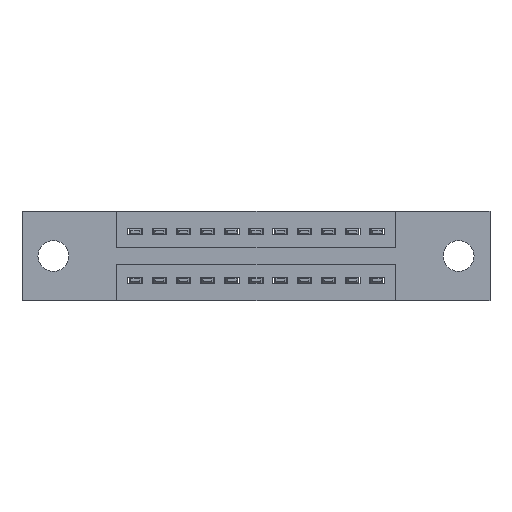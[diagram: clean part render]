
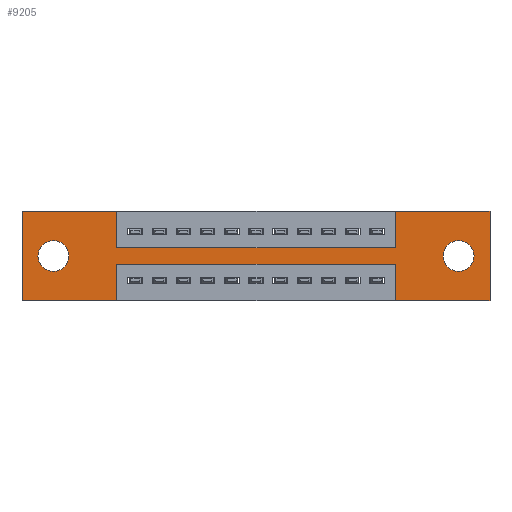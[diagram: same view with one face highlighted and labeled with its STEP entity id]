
A CAD part, front view. The second image highlights one B-rep face of the part: STEP entity #9205.
In plain terms, the highlighted planar face has unit normal (0, -1, 0).
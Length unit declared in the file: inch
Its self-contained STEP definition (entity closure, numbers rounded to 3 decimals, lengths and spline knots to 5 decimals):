
#7 = ORIENTED_EDGE ( 'NONE', *, *, #1507, .F. ) ;
#96 = CARTESIAN_POINT ( 'NONE',  ( 1.5425, 0., -0.15 ) ) ;
#225 = DIRECTION ( 'NONE',  ( 0., 0., 1. ) ) ;
#337 = ORIENTED_EDGE ( 'NONE', *, *, #2822, .F. ) ;
#346 = VECTOR ( 'NONE', #6573, 39.37008 ) ;
#505 = VERTEX_POINT ( 'NONE', #96 ) ;
#539 = VERTEX_POINT ( 'NONE', #2170 ) ;
#620 = FACE_BOUND ( 'NONE', #1701, .T. ) ;
#714 = EDGE_CURVE ( 'NONE', #5986, #6882, #4839, .T. ) ;
#729 = CARTESIAN_POINT ( 'NONE',  ( 0.3925, 0., -0.22 ) ) ;
#983 = CIRCLE ( 'NONE', #7035, 0.064 ) ;
#1058 = CARTESIAN_POINT ( 'NONE',  ( 0.13, 0., -0.121 ) ) ;
#1203 = EDGE_CURVE ( 'NONE', #8654, #8650, #11434, .T. ) ;
#1286 = LINE ( 'NONE', #7946, #9013 ) ;
#1308 = CARTESIAN_POINT ( 'NONE',  ( 0., 0., 0. ) ) ;
#1486 = ORIENTED_EDGE ( 'NONE', *, *, #12150, .T. ) ;
#1507 = EDGE_CURVE ( 'NONE', #6882, #12163, #9912, .T. ) ;
#1580 = LINE ( 'NONE', #7651, #9550 ) ;
#1701 = EDGE_LOOP ( 'NONE', ( #8888, #11293 ) ) ;
#1753 = DIRECTION ( 'NONE',  ( 0., 0., -1. ) ) ;
#1786 = DIRECTION ( 'NONE',  ( 0., 1., 0. ) ) ;
#1807 = ORIENTED_EDGE ( 'NONE', *, *, #4567, .F. ) ;
#1813 = CARTESIAN_POINT ( 'NONE',  ( 1.805, 0., -0.185 ) ) ;
#1900 = LINE ( 'NONE', #4996, #11638 ) ;
#2051 = EDGE_CURVE ( 'NONE', #10428, #4783, #983, .T. ) ;
#2081 = PLANE ( 'NONE',  #5947 ) ;
#2170 = CARTESIAN_POINT ( 'NONE',  ( 1.935, 0., -0.37 ) ) ;
#2176 = CARTESIAN_POINT ( 'NONE',  ( 0., 0., 0. ) ) ;
#2319 = EDGE_CURVE ( 'NONE', #4783, #10428, #12520, .T. ) ;
#2371 = VERTEX_POINT ( 'NONE', #729 ) ;
#2412 = DIRECTION ( 'NONE',  ( 0., 0., -1. ) ) ;
#2484 = ORIENTED_EDGE ( 'NONE', *, *, #10534, .F. ) ;
#2776 = DIRECTION ( 'NONE',  ( 1., 0., 0. ) ) ;
#2822 = EDGE_CURVE ( 'NONE', #8650, #5986, #1286, .T. ) ;
#3068 = VERTEX_POINT ( 'NONE', #11318 ) ;
#3094 = DIRECTION ( 'NONE',  ( 0., 0., -1. ) ) ;
#3098 = ORIENTED_EDGE ( 'NONE', *, *, #1203, .F. ) ;
#3137 = AXIS2_PLACEMENT_3D ( 'NONE', #1813, #1786, #1753 ) ;
#3365 = FACE_OUTER_BOUND ( 'NONE', #4482, .T. ) ;
#3440 = LINE ( 'NONE', #6482, #6171 ) ;
#3688 = VECTOR ( 'NONE', #7209, 39.37008 ) ;
#3947 = EDGE_CURVE ( 'NONE', #7504, #2371, #1580, .T. ) ;
#4091 = DIRECTION ( 'NONE',  ( 1., 0., 0. ) ) ;
#4112 = CIRCLE ( 'NONE', #5354, 0.064 ) ;
#4198 = EDGE_CURVE ( 'NONE', #11257, #7093, #8990, .T. ) ;
#4236 = ORIENTED_EDGE ( 'NONE', *, *, #4198, .T. ) ;
#4347 = CARTESIAN_POINT ( 'NONE',  ( 0.3925, 0., -0.15 ) ) ;
#4482 = EDGE_LOOP ( 'NONE', ( #1807, #7203, #9763, #12130, #7502, #10056, #2484, #5185, #7, #8135, #337, #3098 ) ) ;
#4567 = EDGE_CURVE ( 'NONE', #2371, #8654, #12482, .T. ) ;
#4783 = VERTEX_POINT ( 'NONE', #8374 ) ;
#4839 = LINE ( 'NONE', #8570, #9743 ) ;
#4959 = VECTOR ( 'NONE', #10733, 39.37008 ) ;
#4996 = CARTESIAN_POINT ( 'NONE',  ( 1.5425, 0., 0. ) ) ;
#4997 = VECTOR ( 'NONE', #11927, 39.37008 ) ;
#5185 = ORIENTED_EDGE ( 'NONE', *, *, #11343, .F. ) ;
#5297 = CARTESIAN_POINT ( 'NONE',  ( 0.3925, 0., -0.37 ) ) ;
#5317 = LINE ( 'NONE', #9259, #4997 ) ;
#5354 = AXIS2_PLACEMENT_3D ( 'NONE', #11976, #6372, #225 ) ;
#5770 = CARTESIAN_POINT ( 'NONE',  ( 1.5425, 0., -0.22 ) ) ;
#5947 = AXIS2_PLACEMENT_3D ( 'NONE', #6132, #9085, #3094 ) ;
#5986 = VERTEX_POINT ( 'NONE', #1308 ) ;
#6001 = CARTESIAN_POINT ( 'NONE',  ( 0.13, 0., -0.249 ) ) ;
#6037 = EDGE_CURVE ( 'NONE', #3068, #539, #9807, .T. ) ;
#6096 = FACE_BOUND ( 'NONE', #10351, .T. ) ;
#6132 = CARTESIAN_POINT ( 'NONE',  ( 0., 0., -0.37 ) ) ;
#6171 = VECTOR ( 'NONE', #11282, 39.37008 ) ;
#6372 = DIRECTION ( 'NONE',  ( 0., 1., 0. ) ) ;
#6482 = CARTESIAN_POINT ( 'NONE',  ( 1.5425, 0., -0.37 ) ) ;
#6573 = DIRECTION ( 'NONE',  ( -1., 0., 0. ) ) ;
#6882 = VERTEX_POINT ( 'NONE', #10654 ) ;
#7035 = AXIS2_PLACEMENT_3D ( 'NONE', #11490, #11443, #11372 ) ;
#7093 = VERTEX_POINT ( 'NONE', #1058 ) ;
#7203 = ORIENTED_EDGE ( 'NONE', *, *, #3947, .F. ) ;
#7209 = DIRECTION ( 'NONE',  ( 1., 0., 0. ) ) ;
#7250 = VECTOR ( 'NONE', #8480, 39.37008 ) ;
#7328 = CARTESIAN_POINT ( 'NONE',  ( 0.3925, 0., 0. ) ) ;
#7463 = CARTESIAN_POINT ( 'NONE',  ( 1.935, 0., 0. ) ) ;
#7502 = ORIENTED_EDGE ( 'NONE', *, *, #6037, .F. ) ;
#7504 = VERTEX_POINT ( 'NONE', #5770 ) ;
#7651 = CARTESIAN_POINT ( 'NONE',  ( 0.3925, 0., -0.22 ) ) ;
#7710 = DIRECTION ( 'NONE',  ( -1., 0., 0. ) ) ;
#7900 = EDGE_CURVE ( 'NONE', #539, #9776, #5317, .T. ) ;
#7946 = CARTESIAN_POINT ( 'NONE',  ( 0., 0., 0. ) ) ;
#8085 = LINE ( 'NONE', #2176, #3688 ) ;
#8135 = ORIENTED_EDGE ( 'NONE', *, *, #714, .F. ) ;
#8374 = CARTESIAN_POINT ( 'NONE',  ( 1.805, 0., -0.249 ) ) ;
#8480 = DIRECTION ( 'NONE',  ( 0., 0., -1. ) ) ;
#8570 = CARTESIAN_POINT ( 'NONE',  ( 0., 0., 0. ) ) ;
#8598 = EDGE_CURVE ( 'NONE', #10184, #3068, #8085, .T. ) ;
#8650 = VERTEX_POINT ( 'NONE', #11011 ) ;
#8654 = VERTEX_POINT ( 'NONE', #5297 ) ;
#8778 = CARTESIAN_POINT ( 'NONE',  ( 1.5425, 0., -0.37 ) ) ;
#8888 = ORIENTED_EDGE ( 'NONE', *, *, #2051, .T. ) ;
#8942 = AXIS2_PLACEMENT_3D ( 'NONE', #12438, #12423, #12398 ) ;
#8990 = CIRCLE ( 'NONE', #8942, 0.064 ) ;
#9013 = VECTOR ( 'NONE', #11468, 39.37008 ) ;
#9042 = CARTESIAN_POINT ( 'NONE',  ( 0.3925, 0., -0.15 ) ) ;
#9085 = DIRECTION ( 'NONE',  ( 0., -1., 0. ) ) ;
#9205 = ADVANCED_FACE ( 'NONE', ( #620, #6096, #3365 ), #2081, .T. ) ;
#9259 = CARTESIAN_POINT ( 'NONE',  ( 0., 0., -0.37 ) ) ;
#9310 = CARTESIAN_POINT ( 'NONE',  ( 0., 0., -0.37 ) ) ;
#9384 = CARTESIAN_POINT ( 'NONE',  ( 1.5425, 0., 0. ) ) ;
#9550 = VECTOR ( 'NONE', #7710, 39.37008 ) ;
#9743 = VECTOR ( 'NONE', #2776, 39.37008 ) ;
#9763 = ORIENTED_EDGE ( 'NONE', *, *, #12252, .F. ) ;
#9776 = VERTEX_POINT ( 'NONE', #8778 ) ;
#9783 = CARTESIAN_POINT ( 'NONE',  ( 1.805, 0., -0.121 ) ) ;
#9807 = LINE ( 'NONE', #7463, #7250 ) ;
#9901 = DIRECTION ( 'NONE',  ( 0., 0., 1. ) ) ;
#9912 = LINE ( 'NONE', #7328, #11995 ) ;
#10056 = ORIENTED_EDGE ( 'NONE', *, *, #8598, .F. ) ;
#10113 = VECTOR ( 'NONE', #4091, 39.37008 ) ;
#10184 = VERTEX_POINT ( 'NONE', #9384 ) ;
#10351 = EDGE_LOOP ( 'NONE', ( #1486, #4236 ) ) ;
#10428 = VERTEX_POINT ( 'NONE', #9783 ) ;
#10534 = EDGE_CURVE ( 'NONE', #505, #10184, #1900, .T. ) ;
#10591 = CARTESIAN_POINT ( 'NONE',  ( 0.3925, 0., -0.37 ) ) ;
#10654 = CARTESIAN_POINT ( 'NONE',  ( 0.3925, 0., 0. ) ) ;
#10733 = DIRECTION ( 'NONE',  ( 0., 0., -1. ) ) ;
#11011 = CARTESIAN_POINT ( 'NONE',  ( 0., 0., -0.37 ) ) ;
#11257 = VERTEX_POINT ( 'NONE', #6001 ) ;
#11282 = DIRECTION ( 'NONE',  ( 0., 0., 1. ) ) ;
#11293 = ORIENTED_EDGE ( 'NONE', *, *, #2319, .T. ) ;
#11318 = CARTESIAN_POINT ( 'NONE',  ( 1.935, 0., 0. ) ) ;
#11343 = EDGE_CURVE ( 'NONE', #12163, #505, #12453, .T. ) ;
#11372 = DIRECTION ( 'NONE',  ( 0., 0., -1. ) ) ;
#11434 = LINE ( 'NONE', #9310, #346 ) ;
#11443 = DIRECTION ( 'NONE',  ( 0., 1., 0. ) ) ;
#11468 = DIRECTION ( 'NONE',  ( 0., 0., 1. ) ) ;
#11490 = CARTESIAN_POINT ( 'NONE',  ( 1.805, 0., -0.185 ) ) ;
#11638 = VECTOR ( 'NONE', #9901, 39.37008 ) ;
#11927 = DIRECTION ( 'NONE',  ( -1., 0., 0. ) ) ;
#11976 = CARTESIAN_POINT ( 'NONE',  ( 0.13, 0., -0.185 ) ) ;
#11995 = VECTOR ( 'NONE', #2412, 39.37008 ) ;
#12130 = ORIENTED_EDGE ( 'NONE', *, *, #7900, .F. ) ;
#12150 = EDGE_CURVE ( 'NONE', #7093, #11257, #4112, .T. ) ;
#12163 = VERTEX_POINT ( 'NONE', #4347 ) ;
#12252 = EDGE_CURVE ( 'NONE', #9776, #7504, #3440, .T. ) ;
#12398 = DIRECTION ( 'NONE',  ( 0., 0., 1. ) ) ;
#12423 = DIRECTION ( 'NONE',  ( 0., 1., 0. ) ) ;
#12438 = CARTESIAN_POINT ( 'NONE',  ( 0.13, 0., -0.185 ) ) ;
#12453 = LINE ( 'NONE', #9042, #10113 ) ;
#12482 = LINE ( 'NONE', #10591, #4959 ) ;
#12520 = CIRCLE ( 'NONE', #3137, 0.064 ) ;
